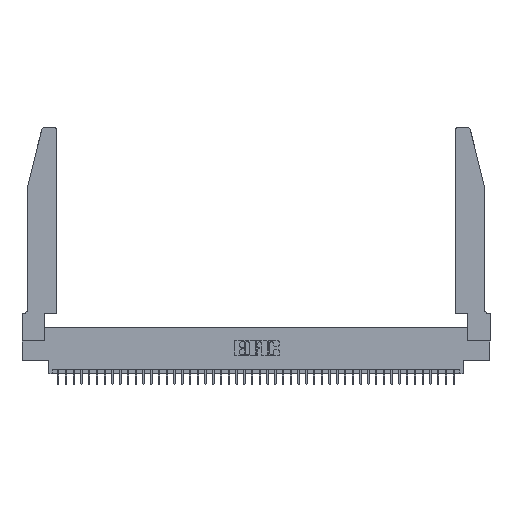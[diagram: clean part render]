
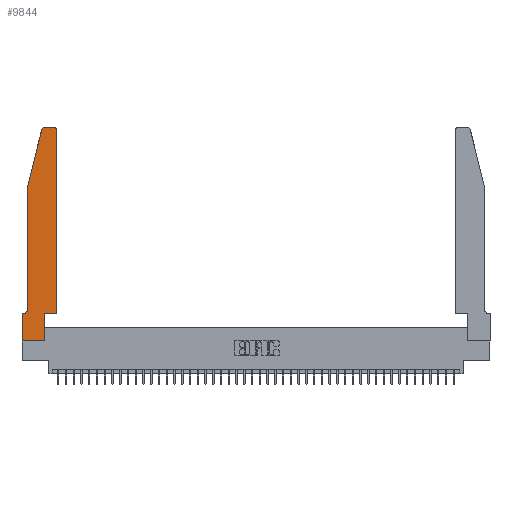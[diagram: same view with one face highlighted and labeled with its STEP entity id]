
A CAD part, top view. The second image highlights one B-rep face of the part: STEP entity #9844.
In plain terms, the highlighted planar face has unit normal (0, 0, 1).
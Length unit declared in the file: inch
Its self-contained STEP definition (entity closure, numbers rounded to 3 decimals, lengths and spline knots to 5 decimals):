
#870 = DIRECTION ( 'NONE',  ( 1., 0., 0. ) ) ;
#1060 = LINE ( 'NONE', #39528, #25565 ) ;
#1895 = CARTESIAN_POINT ( 'NONE',  ( 0.4505, 0.35, 0.37 ) ) ;
#2031 = VECTOR ( 'NONE', #12808, 39.37008 ) ;
#2324 = ORIENTED_EDGE ( 'NONE', *, *, #41694, .T. ) ;
#2601 = VERTEX_POINT ( 'NONE', #36191 ) ;
#2661 = VECTOR ( 'NONE', #15987, 39.37008 ) ;
#2721 = DIRECTION ( 'NONE',  ( -1., 0., 0. ) ) ;
#2763 = VECTOR ( 'NONE', #2721, 39.37008 ) ;
#3169 = CARTESIAN_POINT ( 'NONE',  ( 0.25487, 2.72718, 0.37 ) ) ;
#5173 = LINE ( 'NONE', #43631, #2031 ) ;
#5277 = EDGE_CURVE ( 'NONE', #23382, #41004, #5173, .T. ) ;
#5364 = VERTEX_POINT ( 'NONE', #9664 ) ;
#7089 = DIRECTION ( 'NONE',  ( 1., 0., 0. ) ) ;
#7405 = CARTESIAN_POINT ( 'NONE',  ( 0.4205, 2.72, 0.37 ) ) ;
#8269 = DIRECTION ( 'NONE',  ( 0., -1., 0. ) ) ;
#9319 = CARTESIAN_POINT ( 'NONE',  ( 0.0755, 0.42, 0.37 ) ) ;
#9349 = EDGE_LOOP ( 'NONE', ( #22401, #31086, #28156, #2324, #26120, #31549, #20968, #29950, #27607, #9681, #21761, #12908 ) ) ;
#9664 = CARTESIAN_POINT ( 'NONE',  ( 0.4505, 2.72, 0.37 ) ) ;
#9681 = ORIENTED_EDGE ( 'NONE', *, *, #34349, .T. ) ;
#9844 = ADVANCED_FACE ( 'NONE', ( #41920 ), #35419, .T. ) ;
#9886 = CARTESIAN_POINT ( 'NONE',  ( 0.0755, 2., 0.37 ) ) ;
#10141 = VERTEX_POINT ( 'NONE', #37794 ) ;
#10294 = VERTEX_POINT ( 'NONE', #33061 ) ;
#11779 = VECTOR ( 'NONE', #41400, 39.37008 ) ;
#12808 = DIRECTION ( 'NONE',  ( -0.239, -0.971, 0. ) ) ;
#12908 = ORIENTED_EDGE ( 'NONE', *, *, #32590, .T. ) ;
#13147 = DIRECTION ( 'NONE',  ( 0., 0., 1. ) ) ;
#13286 = CARTESIAN_POINT ( 'NONE',  ( 0.4505, 0.35, 0.37 ) ) ;
#13891 = EDGE_CURVE ( 'NONE', #26390, #29197, #40698, .T. ) ;
#13921 = CARTESIAN_POINT ( 'NONE',  ( 0.2605, 2.75, 0.37 ) ) ;
#15987 = DIRECTION ( 'NONE',  ( 0., -1., 0. ) ) ;
#17584 = CARTESIAN_POINT ( 'NONE',  ( 0.0755, 2., 0.37 ) ) ;
#18773 = VERTEX_POINT ( 'NONE', #13286 ) ;
#18796 = LINE ( 'NONE', #42140, #21343 ) ;
#19438 = EDGE_CURVE ( 'NONE', #2601, #10294, #1060, .T. ) ;
#19672 = LINE ( 'NONE', #30030, #2763 ) ;
#19741 = EDGE_CURVE ( 'NONE', #10294, #36809, #24463, .T. ) ;
#20645 = CARTESIAN_POINT ( 'NONE',  ( 0., 0., 0.37 ) ) ;
#20726 = AXIS2_PLACEMENT_3D ( 'NONE', #41129, #26779, #40469 ) ;
#20810 = EDGE_CURVE ( 'NONE', #36809, #31639, #18796, .T. ) ;
#20968 = ORIENTED_EDGE ( 'NONE', *, *, #19438, .T. ) ;
#21043 = CARTESIAN_POINT ( 'NONE',  ( 0., 0.35, 0.37 ) ) ;
#21132 = CARTESIAN_POINT ( 'NONE',  ( 0.2865, 0.35, 0.37 ) ) ;
#21343 = VECTOR ( 'NONE', #29139, 39.37008 ) ;
#21524 = CIRCLE ( 'NONE', #39453, 0.03 ) ;
#21761 = ORIENTED_EDGE ( 'NONE', *, *, #26510, .T. ) ;
#22401 = ORIENTED_EDGE ( 'NONE', *, *, #13891, .T. ) ;
#23382 = VERTEX_POINT ( 'NONE', #3169 ) ;
#24428 = DIRECTION ( 'NONE',  ( 0., 0., 1. ) ) ;
#24463 = LINE ( 'NONE', #20645, #27729 ) ;
#25565 = VECTOR ( 'NONE', #8269, 39.37008 ) ;
#26029 = LINE ( 'NONE', #1895, #27104 ) ;
#26120 = ORIENTED_EDGE ( 'NONE', *, *, #33737, .T. ) ;
#26390 = VERTEX_POINT ( 'NONE', #29802 ) ;
#26416 = CIRCLE ( 'NONE', #42208, 0.03 ) ;
#26510 = EDGE_CURVE ( 'NONE', #18773, #5364, #41177, .T. ) ;
#26779 = DIRECTION ( 'NONE',  ( 0., 0., -1. ) ) ;
#27104 = VECTOR ( 'NONE', #29198, 39.37008 ) ;
#27461 = DIRECTION ( 'NONE',  ( -1., 0., 0. ) ) ;
#27607 = ORIENTED_EDGE ( 'NONE', *, *, #20810, .T. ) ;
#27729 = VECTOR ( 'NONE', #7089, 39.37008 ) ;
#28156 = ORIENTED_EDGE ( 'NONE', *, *, #5277, .T. ) ;
#29139 = DIRECTION ( 'NONE',  ( 0., 1., 0. ) ) ;
#29197 = VERTEX_POINT ( 'NONE', #36768 ) ;
#29198 = DIRECTION ( 'NONE',  ( 1., 0., 0. ) ) ;
#29656 = VECTOR ( 'NONE', #27461, 39.37008 ) ;
#29802 = CARTESIAN_POINT ( 'NONE',  ( 0.4205, 2.75, 0.37 ) ) ;
#29950 = ORIENTED_EDGE ( 'NONE', *, *, #19741, .T. ) ;
#29968 = LINE ( 'NONE', #9886, #2661 ) ;
#30030 = CARTESIAN_POINT ( 'NONE',  ( 0.0755, 0.35, 0.37 ) ) ;
#31086 = ORIENTED_EDGE ( 'NONE', *, *, #44052, .T. ) ;
#31100 = CARTESIAN_POINT ( 'NONE',  ( 0.4505, 0.35, 0.37 ) ) ;
#31502 = CIRCLE ( 'NONE', #20726, 0.07 ) ;
#31549 = ORIENTED_EDGE ( 'NONE', *, *, #36240, .T. ) ;
#31639 = VERTEX_POINT ( 'NONE', #21132 ) ;
#32590 = EDGE_CURVE ( 'NONE', #5364, #26390, #26416, .T. ) ;
#33061 = CARTESIAN_POINT ( 'NONE',  ( 0., 0., 0.37 ) ) ;
#33436 = CARTESIAN_POINT ( 'NONE',  ( 0.284, 2.72, 0.37 ) ) ;
#33737 = EDGE_CURVE ( 'NONE', #35656, #10141, #31502, .T. ) ;
#33759 = CARTESIAN_POINT ( 'NONE',  ( 0.2865, 0., 0.37 ) ) ;
#33867 = DIRECTION ( 'NONE',  ( 1., 0., 0. ) ) ;
#34349 = EDGE_CURVE ( 'NONE', #31639, #18773, #26029, .T. ) ;
#34890 = DIRECTION ( 'NONE',  ( 0., 0., 1. ) ) ;
#35419 = PLANE ( 'NONE',  #40246 ) ;
#35656 = VERTEX_POINT ( 'NONE', #9319 ) ;
#36191 = CARTESIAN_POINT ( 'NONE',  ( 0., 0.35, 0.37 ) ) ;
#36240 = EDGE_CURVE ( 'NONE', #10141, #2601, #19672, .T. ) ;
#36768 = CARTESIAN_POINT ( 'NONE',  ( 0.284, 2.75, 0.37 ) ) ;
#36809 = VERTEX_POINT ( 'NONE', #33759 ) ;
#37794 = CARTESIAN_POINT ( 'NONE',  ( 0.0055, 0.35, 0.37 ) ) ;
#39453 = AXIS2_PLACEMENT_3D ( 'NONE', #33436, #13147, #33867 ) ;
#39528 = CARTESIAN_POINT ( 'NONE',  ( 0., 0., 0.37 ) ) ;
#40246 = AXIS2_PLACEMENT_3D ( 'NONE', #21043, #24428, #42377 ) ;
#40469 = DIRECTION ( 'NONE',  ( -1., 0., 0. ) ) ;
#40698 = LINE ( 'NONE', #13921, #29656 ) ;
#41004 = VERTEX_POINT ( 'NONE', #17584 ) ;
#41129 = CARTESIAN_POINT ( 'NONE',  ( 0.0055, 0.42, 0.37 ) ) ;
#41177 = LINE ( 'NONE', #31100, #11779 ) ;
#41400 = DIRECTION ( 'NONE',  ( 0., 1., 0. ) ) ;
#41694 = EDGE_CURVE ( 'NONE', #41004, #35656, #29968, .T. ) ;
#41920 = FACE_OUTER_BOUND ( 'NONE', #9349, .T. ) ;
#42140 = CARTESIAN_POINT ( 'NONE',  ( 0.2865, 0.35, 0.37 ) ) ;
#42208 = AXIS2_PLACEMENT_3D ( 'NONE', #7405, #34890, #870 ) ;
#42377 = DIRECTION ( 'NONE',  ( 1., 0., 0. ) ) ;
#43631 = CARTESIAN_POINT ( 'NONE',  ( 0.0755, 2., 0.37 ) ) ;
#44052 = EDGE_CURVE ( 'NONE', #29197, #23382, #21524, .T. ) ;
